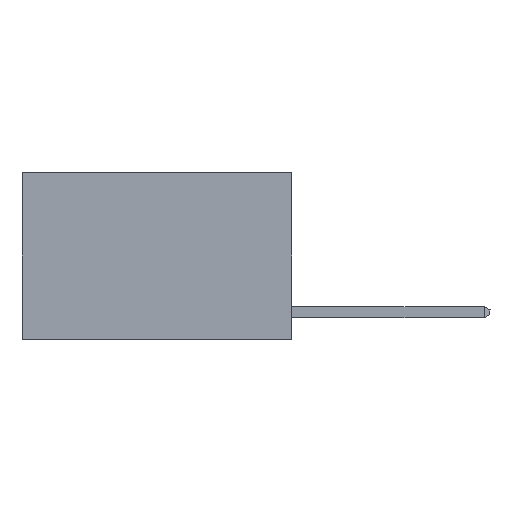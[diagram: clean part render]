
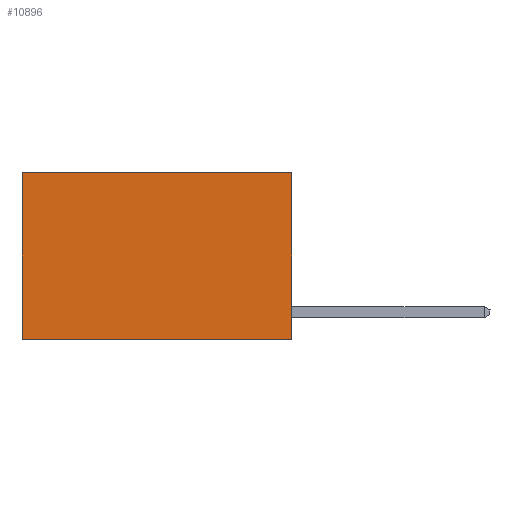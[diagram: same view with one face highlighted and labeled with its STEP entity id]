
A CAD part, left-side view. The second image highlights one B-rep face of the part: STEP entity #10896.
In plain terms, the highlighted planar face has unit normal (-1, 0, 0).
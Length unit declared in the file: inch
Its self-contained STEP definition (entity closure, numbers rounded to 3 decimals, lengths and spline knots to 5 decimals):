
#421 = CARTESIAN_POINT ( 'NONE',  ( 0.2625, 0., 0. ) ) ;
#708 = DIRECTION ( 'NONE',  ( 0., 0., -1. ) ) ;
#872 = VERTEX_POINT ( 'NONE', #3709 ) ;
#2735 = CARTESIAN_POINT ( 'NONE',  ( 0.2625, 0.6, -0.37 ) ) ;
#3709 = CARTESIAN_POINT ( 'NONE',  ( 0.2625, 0., 0. ) ) ;
#5154 = LINE ( 'NONE', #6865, #17724 ) ;
#5741 = ORIENTED_EDGE ( 'NONE', *, *, #19424, .F. ) ;
#5867 = DIRECTION ( 'NONE',  ( 0., 0., -1. ) ) ;
#6865 = CARTESIAN_POINT ( 'NONE',  ( 0.2625, 0.6, 0. ) ) ;
#6867 = CARTESIAN_POINT ( 'NONE',  ( 0.2625, 0., 0. ) ) ;
#7123 = VERTEX_POINT ( 'NONE', #19345 ) ;
#7261 = LINE ( 'NONE', #421, #16600 ) ;
#7350 = DIRECTION ( 'NONE',  ( 0., 1., 0. ) ) ;
#8366 = DIRECTION ( 'NONE',  ( 0., 0., -1. ) ) ;
#8452 = DIRECTION ( 'NONE',  ( 1., 0., 0. ) ) ;
#9210 = VERTEX_POINT ( 'NONE', #2735 ) ;
#9291 = VECTOR ( 'NONE', #8366, 39.37008 ) ;
#10020 = LINE ( 'NONE', #16454, #9291 ) ;
#10896 = ADVANCED_FACE ( 'NONE', ( #18452 ), #19404, .F. ) ;
#11994 = EDGE_CURVE ( 'NONE', #16748, #9210, #14971, .T. ) ;
#12245 = CARTESIAN_POINT ( 'NONE',  ( 0.2625, 0., -0.37 ) ) ;
#14029 = ORIENTED_EDGE ( 'NONE', *, *, #11994, .F. ) ;
#14141 = ORIENTED_EDGE ( 'NONE', *, *, #14734, .T. ) ;
#14332 = EDGE_LOOP ( 'NONE', ( #14925, #14029, #5741, #14141 ) ) ;
#14734 = EDGE_CURVE ( 'NONE', #872, #7123, #7261, .T. ) ;
#14771 = DIRECTION ( 'NONE',  ( 0., 1., 0. ) ) ;
#14925 = ORIENTED_EDGE ( 'NONE', *, *, #17784, .T. ) ;
#14971 = LINE ( 'NONE', #12245, #15696 ) ;
#15451 = AXIS2_PLACEMENT_3D ( 'NONE', #6867, #8452, #708 ) ;
#15696 = VECTOR ( 'NONE', #7350, 39.37008 ) ;
#16454 = CARTESIAN_POINT ( 'NONE',  ( 0.2625, 0., 0. ) ) ;
#16600 = VECTOR ( 'NONE', #14771, 39.37008 ) ;
#16748 = VERTEX_POINT ( 'NONE', #19306 ) ;
#17724 = VECTOR ( 'NONE', #5867, 39.37008 ) ;
#17784 = EDGE_CURVE ( 'NONE', #7123, #9210, #5154, .T. ) ;
#18452 = FACE_OUTER_BOUND ( 'NONE', #14332, .T. ) ;
#19306 = CARTESIAN_POINT ( 'NONE',  ( 0.2625, 0., -0.37 ) ) ;
#19345 = CARTESIAN_POINT ( 'NONE',  ( 0.2625, 0.6, 0. ) ) ;
#19404 = PLANE ( 'NONE',  #15451 ) ;
#19424 = EDGE_CURVE ( 'NONE', #872, #16748, #10020, .T. ) ;
